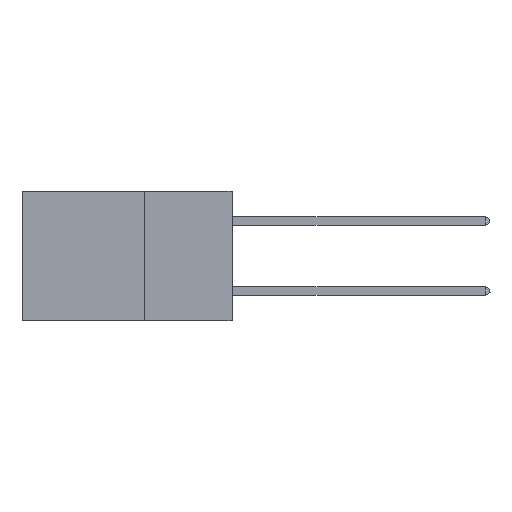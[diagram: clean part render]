
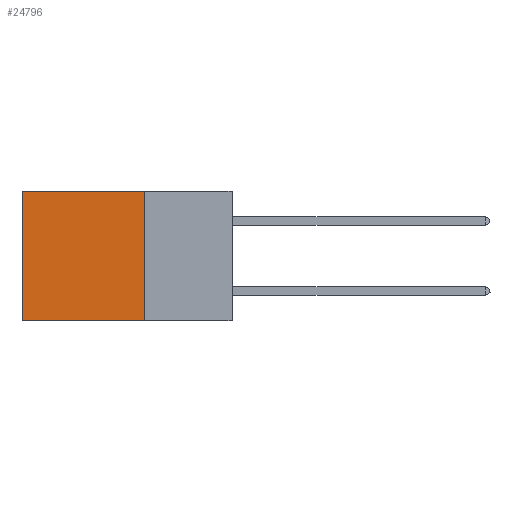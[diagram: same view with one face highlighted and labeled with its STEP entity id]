
A CAD part, left-side view. The second image highlights one B-rep face of the part: STEP entity #24796.
In plain terms, the highlighted planar face has unit normal (-1, 0, 0).
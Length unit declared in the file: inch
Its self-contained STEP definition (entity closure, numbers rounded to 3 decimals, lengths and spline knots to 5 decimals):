
#517 = DIRECTION ( 'NONE',  ( 0., 1., 0. ) ) ;
#1181 = FACE_OUTER_BOUND ( 'NONE', #26474, .T. ) ;
#1615 = CARTESIAN_POINT ( 'NONE',  ( 0.2875, 0.6, 0. ) ) ;
#2486 = ORIENTED_EDGE ( 'NONE', *, *, #31405, .F. ) ;
#5545 = CARTESIAN_POINT ( 'NONE',  ( 0.2875, 0.6, -0.37 ) ) ;
#8125 = DIRECTION ( 'NONE',  ( 0., 0., -1. ) ) ;
#8408 = VERTEX_POINT ( 'NONE', #5545 ) ;
#8553 = EDGE_CURVE ( 'NONE', #29875, #25203, #25479, .T. ) ;
#9118 = CARTESIAN_POINT ( 'NONE',  ( 0.2875, 0.25, 0. ) ) ;
#9377 = LINE ( 'NONE', #22822, #37334 ) ;
#10209 = CARTESIAN_POINT ( 'NONE',  ( 0.2875, 0.25, 0. ) ) ;
#10287 = VECTOR ( 'NONE', #8125, 39.37008 ) ;
#10771 = LINE ( 'NONE', #36620, #10287 ) ;
#12365 = DIRECTION ( 'NONE',  ( 0., 1., 0. ) ) ;
#14328 = EDGE_CURVE ( 'NONE', #25203, #8408, #9377, .T. ) ;
#15596 = EDGE_CURVE ( 'NONE', #27362, #8408, #17359, .T. ) ;
#15655 = DIRECTION ( 'NONE',  ( 1., 0., 0. ) ) ;
#17359 = LINE ( 'NONE', #19959, #30299 ) ;
#19959 = CARTESIAN_POINT ( 'NONE',  ( 0.2875, 0.25, -0.37 ) ) ;
#22822 = CARTESIAN_POINT ( 'NONE',  ( 0.2875, 0.6, 0. ) ) ;
#24796 = ADVANCED_FACE ( 'NONE', ( #1181 ), #24894, .F. ) ;
#24894 = PLANE ( 'NONE',  #30411 ) ;
#25203 = VERTEX_POINT ( 'NONE', #1615 ) ;
#25479 = LINE ( 'NONE', #9118, #32925 ) ;
#26474 = EDGE_LOOP ( 'NONE', ( #38568, #34835, #2486, #27484 ) ) ;
#27362 = VERTEX_POINT ( 'NONE', #30964 ) ;
#27484 = ORIENTED_EDGE ( 'NONE', *, *, #8553, .T. ) ;
#29875 = VERTEX_POINT ( 'NONE', #10209 ) ;
#30299 = VECTOR ( 'NONE', #517, 39.37008 ) ;
#30411 = AXIS2_PLACEMENT_3D ( 'NONE', #37822, #15655, #37969 ) ;
#30964 = CARTESIAN_POINT ( 'NONE',  ( 0.2875, 0.25, -0.37 ) ) ;
#31405 = EDGE_CURVE ( 'NONE', #29875, #27362, #10771, .T. ) ;
#32925 = VECTOR ( 'NONE', #12365, 39.37008 ) ;
#34835 = ORIENTED_EDGE ( 'NONE', *, *, #15596, .F. ) ;
#34986 = DIRECTION ( 'NONE',  ( 0., 0., -1. ) ) ;
#36620 = CARTESIAN_POINT ( 'NONE',  ( 0.2875, 0.25, 0. ) ) ;
#37334 = VECTOR ( 'NONE', #34986, 39.37008 ) ;
#37822 = CARTESIAN_POINT ( 'NONE',  ( 0.2875, 0.25, 0. ) ) ;
#37969 = DIRECTION ( 'NONE',  ( 0., 0., -1. ) ) ;
#38568 = ORIENTED_EDGE ( 'NONE', *, *, #14328, .T. ) ;
